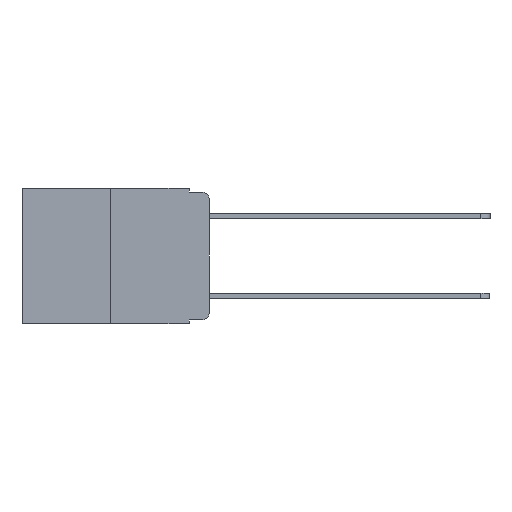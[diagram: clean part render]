
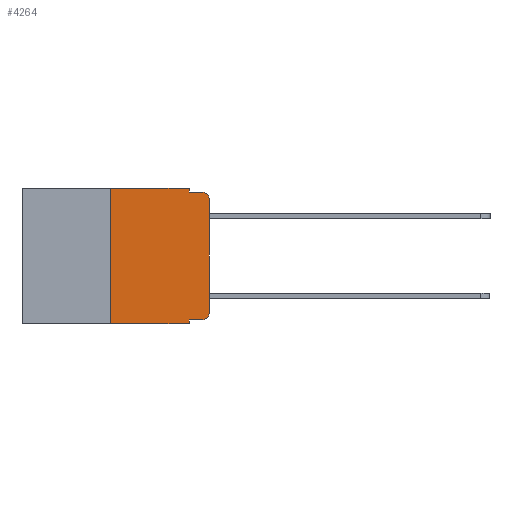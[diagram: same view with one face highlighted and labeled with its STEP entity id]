
A CAD part, left-side view. The second image highlights one B-rep face of the part: STEP entity #4264.
In plain terms, the highlighted planar face has unit normal (-1, 0, 0).
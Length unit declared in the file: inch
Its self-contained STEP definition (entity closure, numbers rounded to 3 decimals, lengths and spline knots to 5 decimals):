
#174 = DIRECTION ( 'NONE',  ( 0., -1., 0. ) ) ;
#225 = LINE ( 'NONE', #3278, #9730 ) ;
#383 = EDGE_CURVE ( 'NONE', #9731, #1624, #6996, .T. ) ;
#616 = VERTEX_POINT ( 'NONE', #8926 ) ;
#691 = EDGE_CURVE ( 'NONE', #10836, #616, #5047, .T. ) ;
#721 = VERTEX_POINT ( 'NONE', #5649 ) ;
#1063 = EDGE_CURVE ( 'NONE', #11314, #11193, #4168, .T. ) ;
#1358 = DIRECTION ( 'NONE',  ( 0., -1., 0. ) ) ;
#1478 = EDGE_CURVE ( 'NONE', #11631, #11314, #2224, .T. ) ;
#1537 = ORIENTED_EDGE ( 'NONE', *, *, #11131, .F. ) ;
#1616 = VECTOR ( 'NONE', #5170, 39.37008 ) ;
#1624 = VERTEX_POINT ( 'NONE', #11534 ) ;
#2096 = DIRECTION ( 'NONE',  ( 0., 0., -1. ) ) ;
#2132 = VECTOR ( 'NONE', #8801, 39.37008 ) ;
#2224 = LINE ( 'NONE', #7778, #6833 ) ;
#2350 = VERTEX_POINT ( 'NONE', #6146 ) ;
#2479 = EDGE_LOOP ( 'NONE', ( #4563, #6530, #1537, #6425, #6551, #9163, #11612, #5429, #9290, #7320 ) ) ;
#2547 = VECTOR ( 'NONE', #3306, 39.37008 ) ;
#2947 = AXIS2_PLACEMENT_3D ( 'NONE', #4756, #10705, #5671 ) ;
#2972 = DIRECTION ( 'NONE',  ( -1., 0., 0. ) ) ;
#3165 = DIRECTION ( 'NONE',  ( 0., -1., 0. ) ) ;
#3228 = CARTESIAN_POINT ( 'NONE',  ( 0., 0.473, -0.343 ) ) ;
#3278 = CARTESIAN_POINT ( 'NONE',  ( 0., 0.051, -0.01 ) ) ;
#3306 = DIRECTION ( 'NONE',  ( 0., 0., 1. ) ) ;
#4168 = LINE ( 'NONE', #5975, #1616 ) ;
#4264 = ADVANCED_FACE ( 'NONE', ( #10270 ), #6737, .F. ) ;
#4425 = EDGE_CURVE ( 'NONE', #6716, #2350, #4652, .T. ) ;
#4486 = CARTESIAN_POINT ( 'NONE',  ( 0., 0.25, 0. ) ) ;
#4563 = ORIENTED_EDGE ( 'NONE', *, *, #691, .T. ) ;
#4652 = LINE ( 'NONE', #7960, #2132 ) ;
#4675 = CARTESIAN_POINT ( 'NONE',  ( 0., 0.25, 0. ) ) ;
#4753 = AXIS2_PLACEMENT_3D ( 'NONE', #8357, #2972, #9184 ) ;
#4756 = CARTESIAN_POINT ( 'NONE',  ( 0., 0.02, -0.03 ) ) ;
#5047 = LINE ( 'NONE', #7267, #2547 ) ;
#5170 = DIRECTION ( 'NONE',  ( 0., 0., -1. ) ) ;
#5226 = LINE ( 'NONE', #8416, #7295 ) ;
#5301 = CARTESIAN_POINT ( 'NONE',  ( 0., 0.051, -0.333 ) ) ;
#5413 = CIRCLE ( 'NONE', #4753, 0.02 ) ;
#5429 = ORIENTED_EDGE ( 'NONE', *, *, #9690, .F. ) ;
#5649 = CARTESIAN_POINT ( 'NONE',  ( 0., 0.02, -0.01 ) ) ;
#5671 = DIRECTION ( 'NONE',  ( 0., 0., -1. ) ) ;
#5975 = CARTESIAN_POINT ( 'NONE',  ( 0., 0.051, 0. ) ) ;
#6146 = CARTESIAN_POINT ( 'NONE',  ( 0., 0.02, -0.333 ) ) ;
#6330 = LINE ( 'NONE', #4486, #8350 ) ;
#6425 = ORIENTED_EDGE ( 'NONE', *, *, #1063, .F. ) ;
#6530 = ORIENTED_EDGE ( 'NONE', *, *, #11667, .T. ) ;
#6551 = ORIENTED_EDGE ( 'NONE', *, *, #1478, .F. ) ;
#6716 = VERTEX_POINT ( 'NONE', #5301 ) ;
#6737 = PLANE ( 'NONE',  #10577 ) ;
#6833 = VECTOR ( 'NONE', #3165, 39.37008 ) ;
#6996 = LINE ( 'NONE', #3228, #11636 ) ;
#7084 = CARTESIAN_POINT ( 'NONE',  ( 0., 0.473, 0. ) ) ;
#7267 = CARTESIAN_POINT ( 'NONE',  ( 0., 0., 0. ) ) ;
#7295 = VECTOR ( 'NONE', #2096, 39.37008 ) ;
#7320 = ORIENTED_EDGE ( 'NONE', *, *, #7556, .T. ) ;
#7556 = EDGE_CURVE ( 'NONE', #2350, #10836, #5413, .T. ) ;
#7778 = CARTESIAN_POINT ( 'NONE',  ( 0., 0.473, 0. ) ) ;
#7960 = CARTESIAN_POINT ( 'NONE',  ( 0., 0.051, -0.333 ) ) ;
#8350 = VECTOR ( 'NONE', #10472, 39.37008 ) ;
#8357 = CARTESIAN_POINT ( 'NONE',  ( 0., 0.02, -0.313 ) ) ;
#8416 = CARTESIAN_POINT ( 'NONE',  ( 0., 0.051, 0. ) ) ;
#8801 = DIRECTION ( 'NONE',  ( 0., -1., 0. ) ) ;
#8926 = CARTESIAN_POINT ( 'NONE',  ( 0., 0., -0.03 ) ) ;
#9163 = ORIENTED_EDGE ( 'NONE', *, *, #10248, .F. ) ;
#9184 = DIRECTION ( 'NONE',  ( 0., 0., -1. ) ) ;
#9290 = ORIENTED_EDGE ( 'NONE', *, *, #4425, .T. ) ;
#9566 = DIRECTION ( 'NONE',  ( 1., 0., 0. ) ) ;
#9690 = EDGE_CURVE ( 'NONE', #6716, #1624, #5226, .T. ) ;
#9730 = VECTOR ( 'NONE', #1358, 39.37008 ) ;
#9731 = VERTEX_POINT ( 'NONE', #11685 ) ;
#10248 = EDGE_CURVE ( 'NONE', #9731, #11631, #6330, .T. ) ;
#10270 = FACE_OUTER_BOUND ( 'NONE', #2479, .T. ) ;
#10472 = DIRECTION ( 'NONE',  ( 0., 0., 1. ) ) ;
#10577 = AXIS2_PLACEMENT_3D ( 'NONE', #7084, #9566, #11397 ) ;
#10705 = DIRECTION ( 'NONE',  ( -1., 0., 0. ) ) ;
#10750 = CIRCLE ( 'NONE', #2947, 0.02 ) ;
#10836 = VERTEX_POINT ( 'NONE', #11674 ) ;
#11110 = CARTESIAN_POINT ( 'NONE',  ( 0., 0.051, -0.01 ) ) ;
#11131 = EDGE_CURVE ( 'NONE', #11193, #721, #225, .T. ) ;
#11193 = VERTEX_POINT ( 'NONE', #11110 ) ;
#11221 = CARTESIAN_POINT ( 'NONE',  ( 0., 0.051, 0. ) ) ;
#11314 = VERTEX_POINT ( 'NONE', #11221 ) ;
#11397 = DIRECTION ( 'NONE',  ( 0., 0., -1. ) ) ;
#11534 = CARTESIAN_POINT ( 'NONE',  ( 0., 0.051, -0.343 ) ) ;
#11612 = ORIENTED_EDGE ( 'NONE', *, *, #383, .T. ) ;
#11631 = VERTEX_POINT ( 'NONE', #4675 ) ;
#11636 = VECTOR ( 'NONE', #174, 39.37008 ) ;
#11667 = EDGE_CURVE ( 'NONE', #616, #721, #10750, .T. ) ;
#11674 = CARTESIAN_POINT ( 'NONE',  ( 0., 0., -0.313 ) ) ;
#11685 = CARTESIAN_POINT ( 'NONE',  ( 0., 0.25, -0.343 ) ) ;
